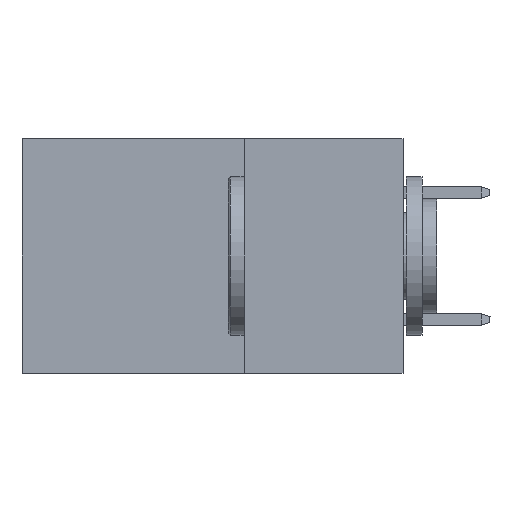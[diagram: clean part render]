
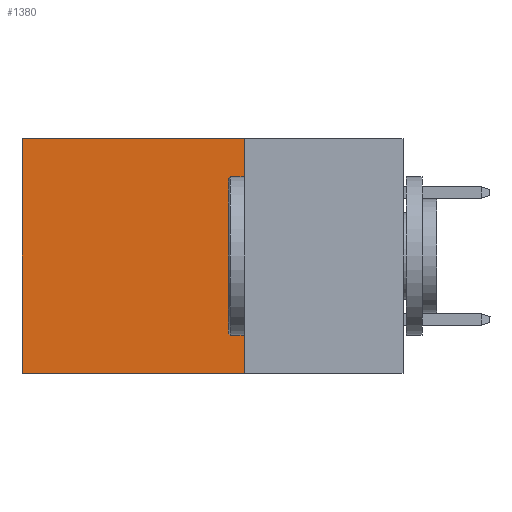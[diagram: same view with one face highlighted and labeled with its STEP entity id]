
A CAD part, left-side view. The second image highlights one B-rep face of the part: STEP entity #1380.
In plain terms, the highlighted planar face has unit normal (-1, 0, 0).
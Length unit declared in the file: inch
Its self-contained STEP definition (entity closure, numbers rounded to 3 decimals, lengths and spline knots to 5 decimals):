
#1380 = ADVANCED_FACE ( 'NONE', ( #5211 ), #16051, .F. ) ;
#2941 = CARTESIAN_POINT ( 'NONE',  ( 0.2875, 0.6, 0. ) ) ;
#3530 = AXIS2_PLACEMENT_3D ( 'NONE', #8035, #28199, #19596 ) ;
#5211 = FACE_OUTER_BOUND ( 'NONE', #29662, .T. ) ;
#6509 = DIRECTION ( 'NONE',  ( 0., 1., 0. ) ) ;
#7702 = VERTEX_POINT ( 'NONE', #9199 ) ;
#7781 = CARTESIAN_POINT ( 'NONE',  ( 0.2875, 0.25, 0. ) ) ;
#8035 = CARTESIAN_POINT ( 'NONE',  ( 0.2875, 0.25, 0. ) ) ;
#9199 = CARTESIAN_POINT ( 'NONE',  ( 0.2875, 0.25, 0. ) ) ;
#9433 = VERTEX_POINT ( 'NONE', #24907 ) ;
#10396 = EDGE_CURVE ( 'NONE', #7702, #9433, #17290, .T. ) ;
#15151 = CARTESIAN_POINT ( 'NONE',  ( 0.2875, 0.6, -0.37 ) ) ;
#16051 = PLANE ( 'NONE',  #3530 ) ;
#16736 = VECTOR ( 'NONE', #30574, 39.37008 ) ;
#17290 = LINE ( 'NONE', #34327, #31008 ) ;
#17719 = LINE ( 'NONE', #29117, #27407 ) ;
#17948 = ORIENTED_EDGE ( 'NONE', *, *, #32960, .T. ) ;
#18337 = ORIENTED_EDGE ( 'NONE', *, *, #10396, .F. ) ;
#19596 = DIRECTION ( 'NONE',  ( 0., 0., -1. ) ) ;
#20094 = DIRECTION ( 'NONE',  ( 0., 0., -1. ) ) ;
#20216 = VECTOR ( 'NONE', #23116, 39.37008 ) ;
#20833 = VERTEX_POINT ( 'NONE', #22591 ) ;
#22591 = CARTESIAN_POINT ( 'NONE',  ( 0.2875, 0.6, 0. ) ) ;
#23116 = DIRECTION ( 'NONE',  ( 0., 0., -1. ) ) ;
#23755 = VERTEX_POINT ( 'NONE', #15151 ) ;
#24073 = ORIENTED_EDGE ( 'NONE', *, *, #32915, .F. ) ;
#24907 = CARTESIAN_POINT ( 'NONE',  ( 0.2875, 0.25, -0.37 ) ) ;
#27407 = VECTOR ( 'NONE', #6509, 39.37008 ) ;
#28199 = DIRECTION ( 'NONE',  ( 1., 0., 0. ) ) ;
#28709 = EDGE_CURVE ( 'NONE', #7702, #20833, #33405, .T. ) ;
#29117 = CARTESIAN_POINT ( 'NONE',  ( 0.2875, 0.25, -0.37 ) ) ;
#29662 = EDGE_LOOP ( 'NONE', ( #17948, #24073, #18337, #32283 ) ) ;
#30574 = DIRECTION ( 'NONE',  ( 0., 1., 0. ) ) ;
#31008 = VECTOR ( 'NONE', #20094, 39.37008 ) ;
#31547 = LINE ( 'NONE', #2941, #20216 ) ;
#32283 = ORIENTED_EDGE ( 'NONE', *, *, #28709, .T. ) ;
#32915 = EDGE_CURVE ( 'NONE', #9433, #23755, #17719, .T. ) ;
#32960 = EDGE_CURVE ( 'NONE', #20833, #23755, #31547, .T. ) ;
#33405 = LINE ( 'NONE', #7781, #16736 ) ;
#34327 = CARTESIAN_POINT ( 'NONE',  ( 0.2875, 0.25, 0. ) ) ;
